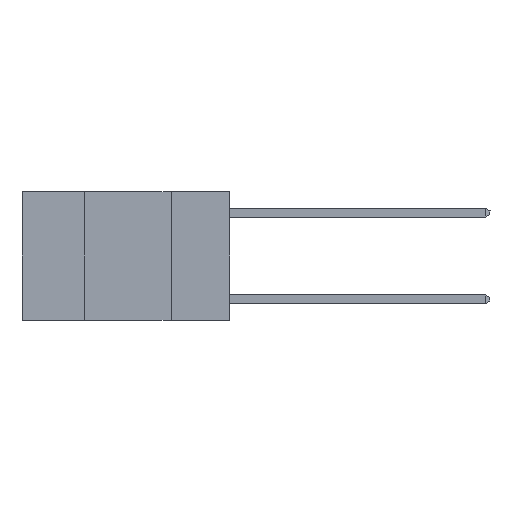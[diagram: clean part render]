
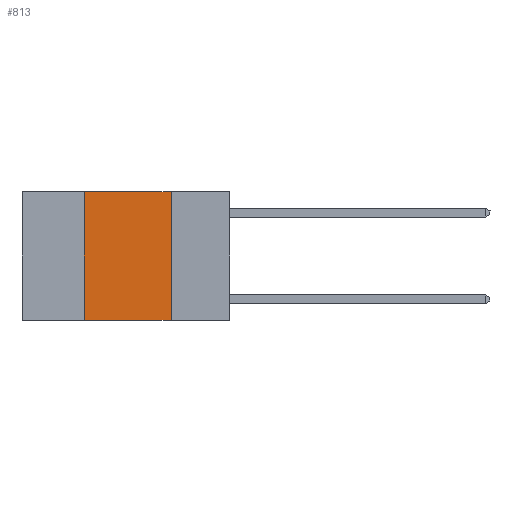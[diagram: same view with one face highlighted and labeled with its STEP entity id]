
A CAD part, left-side view. The second image highlights one B-rep face of the part: STEP entity #813.
In plain terms, the highlighted planar face has unit normal (-1, 0, 0).
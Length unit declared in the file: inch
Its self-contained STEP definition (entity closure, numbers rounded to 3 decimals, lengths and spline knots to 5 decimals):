
#144 = CARTESIAN_POINT ( 'NONE',  ( 0., 0.6, 0. ) ) ;
#220 = EDGE_CURVE ( 'NONE', #7545, #1032, #8653, .T. ) ;
#701 = CARTESIAN_POINT ( 'NONE',  ( 0., 0.42, -0.37 ) ) ;
#792 = DIRECTION ( 'NONE',  ( 0., 0., -1. ) ) ;
#813 = ADVANCED_FACE ( 'NONE', ( #5440 ), #5299, .F. ) ;
#875 = LINE ( 'NONE', #8532, #6724 ) ;
#991 = DIRECTION ( 'NONE',  ( 1., 0., 0. ) ) ;
#1032 = VERTEX_POINT ( 'NONE', #8963 ) ;
#1255 = EDGE_CURVE ( 'NONE', #7827, #1032, #5897, .T. ) ;
#2214 = CARTESIAN_POINT ( 'NONE',  ( 0., 0.6, 0. ) ) ;
#2898 = DIRECTION ( 'NONE',  ( 0., 0., -1. ) ) ;
#3564 = VECTOR ( 'NONE', #6829, 39.37008 ) ;
#3733 = VECTOR ( 'NONE', #2898, 39.37008 ) ;
#3907 = AXIS2_PLACEMENT_3D ( 'NONE', #144, #991, #792 ) ;
#4271 = EDGE_LOOP ( 'NONE', ( #6908, #4677, #8782, #9035 ) ) ;
#4677 = ORIENTED_EDGE ( 'NONE', *, *, #5512, .F. ) ;
#4703 = EDGE_CURVE ( 'NONE', #7827, #6698, #875, .T. ) ;
#4979 = VECTOR ( 'NONE', #6598, 39.37008 ) ;
#5008 = CARTESIAN_POINT ( 'NONE',  ( 0., 0.42, 0. ) ) ;
#5078 = CARTESIAN_POINT ( 'NONE',  ( 0., 0.17, 0. ) ) ;
#5299 = PLANE ( 'NONE',  #3907 ) ;
#5342 = DIRECTION ( 'NONE',  ( 0., 0., 1. ) ) ;
#5440 = FACE_OUTER_BOUND ( 'NONE', #4271, .T. ) ;
#5512 = EDGE_CURVE ( 'NONE', #6698, #7545, #7521, .T. ) ;
#5897 = LINE ( 'NONE', #6540, #4979 ) ;
#6540 = CARTESIAN_POINT ( 'NONE',  ( 0., 0.6, -0.37 ) ) ;
#6598 = DIRECTION ( 'NONE',  ( 0., -1., 0. ) ) ;
#6698 = VERTEX_POINT ( 'NONE', #5008 ) ;
#6724 = VECTOR ( 'NONE', #5342, 39.37008 ) ;
#6829 = DIRECTION ( 'NONE',  ( 0., -1., 0. ) ) ;
#6908 = ORIENTED_EDGE ( 'NONE', *, *, #220, .F. ) ;
#7521 = LINE ( 'NONE', #2214, #3564 ) ;
#7545 = VERTEX_POINT ( 'NONE', #8485 ) ;
#7827 = VERTEX_POINT ( 'NONE', #701 ) ;
#8485 = CARTESIAN_POINT ( 'NONE',  ( 0., 0.17, 0. ) ) ;
#8532 = CARTESIAN_POINT ( 'NONE',  ( 0., 0.42, 0. ) ) ;
#8653 = LINE ( 'NONE', #5078, #3733 ) ;
#8782 = ORIENTED_EDGE ( 'NONE', *, *, #4703, .F. ) ;
#8963 = CARTESIAN_POINT ( 'NONE',  ( 0., 0.17, -0.37 ) ) ;
#9035 = ORIENTED_EDGE ( 'NONE', *, *, #1255, .T. ) ;
